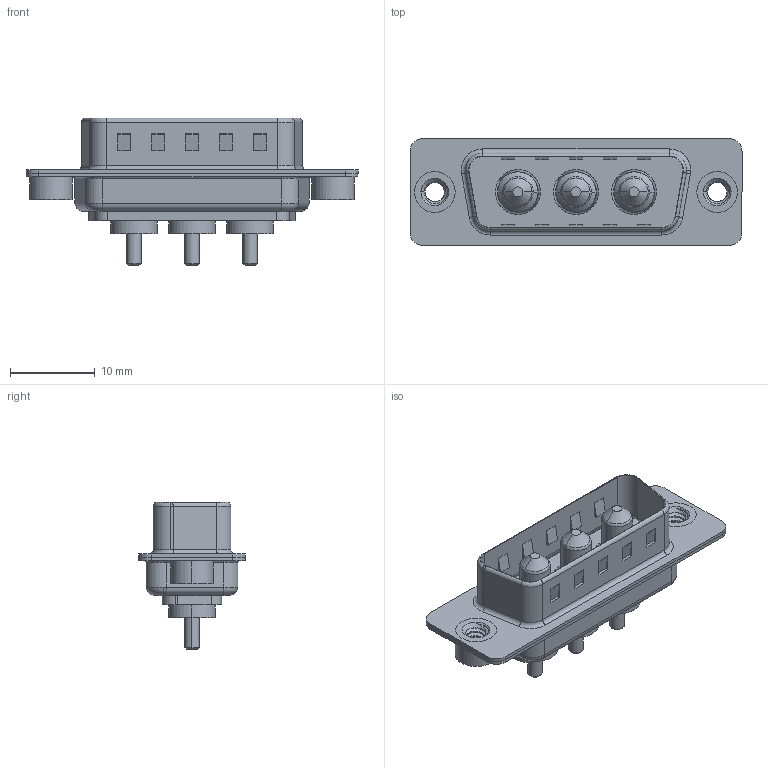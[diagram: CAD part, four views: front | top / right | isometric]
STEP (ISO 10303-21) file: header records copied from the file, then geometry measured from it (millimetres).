
FILE_DESCRIPTION (( 'STEP AP203' ), '1' );
FILE_NAME ('627-3W3-624-1N2.STEP', '2019-05-24T16:43:39', ( '' ), ( '' ), 'SwSTEP 2.0', 'SolidWorks 2016', '' );
FILE_SCHEMA (( 'CONFIG_CONTROL_DESIGN' ));
Length unit declared in the file: millimetre
Products named in the file (6): 627Combo Shell Front_15 Contacts; 627Combo Threaded Rivet_2; Power Pin_10A S; 627-3W3-624-1N2; 627Combo Housing_3W3; 627Combo Shell Rear_15 Contacts
Assembly tree (8 placements, depth 2):
  627-3W3-624-1N2
    627Combo Housing_3W3
    627Combo Shell Rear_15 Contacts
    627Combo Shell Front_15 Contacts
    627Combo Threaded Rivet_2  x2
    Power Pin_10A S  x3
Bounding box: 39.15 x 12.6 x 17.4 mm (x, y, z)
Volume: 2005.2 mm3; surface area: 4668.8 mm2
Topology: 11 solids, 11 shells, 460 faces, 1112 edges, 694 vertices
Faces by surface type: cylinder 190, plane 169, torus 56, cone 33, bspline 12
Entity records: 12798 total; most frequent: CARTESIAN_POINT 3387, DIRECTION 1905, ORIENTED_EDGE 1766, EDGE_CURVE 883, AXIS2_PLACEMENT_3D 710, VERTEX_POINT 554, LINE 485, VECTOR 485
